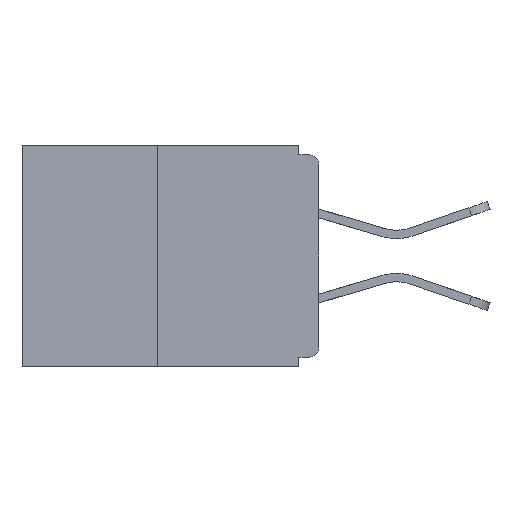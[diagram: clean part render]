
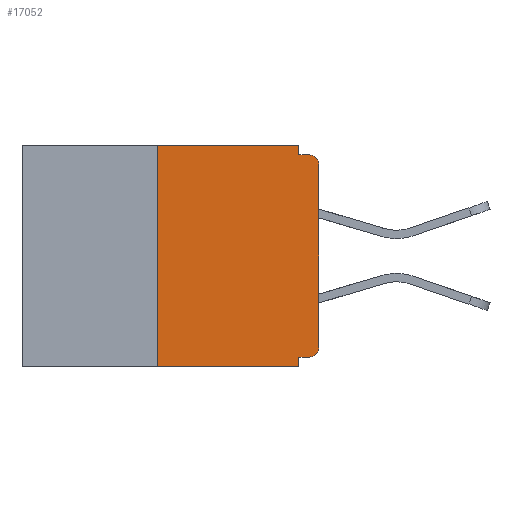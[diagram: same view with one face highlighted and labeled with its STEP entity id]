
A CAD part, left-side view. The second image highlights one B-rep face of the part: STEP entity #17052.
In plain terms, the highlighted planar face has unit normal (-1, 0, 0).
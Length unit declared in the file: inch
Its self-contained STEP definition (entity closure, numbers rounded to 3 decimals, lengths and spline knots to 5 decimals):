
#138 = EDGE_CURVE ( 'NONE', #7621, #7189, #15936, .T. ) ;
#241 = LINE ( 'NONE', #15287, #11779 ) ;
#291 = FACE_OUTER_BOUND ( 'NONE', #16553, .T. ) ;
#328 = CARTESIAN_POINT ( 'NONE',  ( 0., 0.46, -0.343 ) ) ;
#333 = DIRECTION ( 'NONE',  ( 0., 0., 1. ) ) ;
#506 = CIRCLE ( 'NONE', #9485, 0.015 ) ;
#1081 = CARTESIAN_POINT ( 'NONE',  ( 0., 0.46, 0. ) ) ;
#1442 = DIRECTION ( 'NONE',  ( -1., 0., 0. ) ) ;
#1635 = EDGE_CURVE ( 'NONE', #5819, #13735, #7759, .T. ) ;
#1679 = DIRECTION ( 'NONE',  ( 0., 0., -1. ) ) ;
#1821 = LINE ( 'NONE', #14050, #3307 ) ;
#2431 = EDGE_CURVE ( 'NONE', #8469, #7682, #3675, .T. ) ;
#2753 = ORIENTED_EDGE ( 'NONE', *, *, #8613, .T. ) ;
#3055 = CARTESIAN_POINT ( 'NONE',  ( 0., 0.015, -0.015 ) ) ;
#3108 = VECTOR ( 'NONE', #9096, 39.37008 ) ;
#3307 = VECTOR ( 'NONE', #333, 39.37008 ) ;
#3663 = CARTESIAN_POINT ( 'NONE',  ( 0., 0.015, -0.328 ) ) ;
#3675 = LINE ( 'NONE', #1081, #8158 ) ;
#3964 = CARTESIAN_POINT ( 'NONE',  ( 0., 0.031, -0.343 ) ) ;
#5098 = ORIENTED_EDGE ( 'NONE', *, *, #13063, .T. ) ;
#5332 = CARTESIAN_POINT ( 'NONE',  ( 0., 0.031, -0.015 ) ) ;
#5819 = VERTEX_POINT ( 'NONE', #5332 ) ;
#6394 = ORIENTED_EDGE ( 'NONE', *, *, #1635, .F. ) ;
#6465 = CARTESIAN_POINT ( 'NONE',  ( 0., 0.25, 0. ) ) ;
#7095 = DIRECTION ( 'NONE',  ( 0., 0., -1. ) ) ;
#7189 = VERTEX_POINT ( 'NONE', #10118 ) ;
#7287 = DIRECTION ( 'NONE',  ( 0., -1., 0. ) ) ;
#7350 = VERTEX_POINT ( 'NONE', #9395 ) ;
#7621 = VERTEX_POINT ( 'NONE', #3663 ) ;
#7682 = VERTEX_POINT ( 'NONE', #13269 ) ;
#7759 = LINE ( 'NONE', #12800, #9655 ) ;
#8140 = DIRECTION ( 'NONE',  ( 0., 0., -1. ) ) ;
#8158 = VECTOR ( 'NONE', #9282, 39.37008 ) ;
#8469 = VERTEX_POINT ( 'NONE', #6465 ) ;
#8613 = EDGE_CURVE ( 'NONE', #15337, #13735, #506, .T. ) ;
#8953 = ORIENTED_EDGE ( 'NONE', *, *, #14622, .F. ) ;
#9038 = CARTESIAN_POINT ( 'NONE',  ( 0., 0., -0.328 ) ) ;
#9096 = DIRECTION ( 'NONE',  ( 0., 1., 0. ) ) ;
#9282 = DIRECTION ( 'NONE',  ( 0., -1., 0. ) ) ;
#9342 = DIRECTION ( 'NONE',  ( 0., 0., -1. ) ) ;
#9395 = CARTESIAN_POINT ( 'NONE',  ( 0., 0., -0.313 ) ) ;
#9485 = AXIS2_PLACEMENT_3D ( 'NONE', #12541, #1442, #16675 ) ;
#9655 = VECTOR ( 'NONE', #7287, 39.37008 ) ;
#10040 = EDGE_CURVE ( 'NONE', #7682, #5819, #241, .T. ) ;
#10114 = ORIENTED_EDGE ( 'NONE', *, *, #14335, .T. ) ;
#10118 = CARTESIAN_POINT ( 'NONE',  ( 0., 0.031, -0.328 ) ) ;
#10811 = LINE ( 'NONE', #3964, #17464 ) ;
#11029 = VECTOR ( 'NONE', #12617, 39.37008 ) ;
#11166 = PLANE ( 'NONE',  #16465 ) ;
#11359 = CARTESIAN_POINT ( 'NONE',  ( 0., 0.46, 0. ) ) ;
#11487 = VECTOR ( 'NONE', #16562, 39.37008 ) ;
#11779 = VECTOR ( 'NONE', #7095, 39.37008 ) ;
#11919 = LINE ( 'NONE', #13744, #11487 ) ;
#12062 = CARTESIAN_POINT ( 'NONE',  ( 0., 0.015, -0.313 ) ) ;
#12153 = CARTESIAN_POINT ( 'NONE',  ( 0., 0., -0.03 ) ) ;
#12199 = CARTESIAN_POINT ( 'NONE',  ( 0., 0.031, -0.343 ) ) ;
#12541 = CARTESIAN_POINT ( 'NONE',  ( 0., 0.015, -0.03 ) ) ;
#12617 = DIRECTION ( 'NONE',  ( 0., -1., 0. ) ) ;
#12671 = ORIENTED_EDGE ( 'NONE', *, *, #13779, .T. ) ;
#12800 = CARTESIAN_POINT ( 'NONE',  ( 0., 0., -0.015 ) ) ;
#12835 = VERTEX_POINT ( 'NONE', #17239 ) ;
#13063 = EDGE_CURVE ( 'NONE', #7350, #15337, #11919, .T. ) ;
#13256 = VERTEX_POINT ( 'NONE', #12199 ) ;
#13269 = CARTESIAN_POINT ( 'NONE',  ( 0., 0.031, 0. ) ) ;
#13486 = EDGE_CURVE ( 'NONE', #7189, #13256, #10811, .T. ) ;
#13597 = ORIENTED_EDGE ( 'NONE', *, *, #13486, .F. ) ;
#13735 = VERTEX_POINT ( 'NONE', #3055 ) ;
#13744 = CARTESIAN_POINT ( 'NONE',  ( 0., 0., 0. ) ) ;
#13779 = EDGE_CURVE ( 'NONE', #12835, #13256, #16593, .T. ) ;
#14050 = CARTESIAN_POINT ( 'NONE',  ( 0., 0.25, 0. ) ) ;
#14335 = EDGE_CURVE ( 'NONE', #7621, #7350, #17659, .T. ) ;
#14362 = AXIS2_PLACEMENT_3D ( 'NONE', #12062, #16187, #9342 ) ;
#14531 = ORIENTED_EDGE ( 'NONE', *, *, #10040, .F. ) ;
#14622 = EDGE_CURVE ( 'NONE', #12835, #8469, #1821, .T. ) ;
#14850 = ORIENTED_EDGE ( 'NONE', *, *, #2431, .F. ) ;
#15287 = CARTESIAN_POINT ( 'NONE',  ( 0., 0.031, 0. ) ) ;
#15337 = VERTEX_POINT ( 'NONE', #12153 ) ;
#15936 = LINE ( 'NONE', #9038, #3108 ) ;
#16187 = DIRECTION ( 'NONE',  ( -1., 0., 0. ) ) ;
#16465 = AXIS2_PLACEMENT_3D ( 'NONE', #11359, #16734, #1679 ) ;
#16553 = EDGE_LOOP ( 'NONE', ( #14850, #8953, #12671, #13597, #17615, #10114, #5098, #2753, #6394, #14531 ) ) ;
#16562 = DIRECTION ( 'NONE',  ( 0., 0., 1. ) ) ;
#16593 = LINE ( 'NONE', #328, #11029 ) ;
#16675 = DIRECTION ( 'NONE',  ( 0., 0., -1. ) ) ;
#16734 = DIRECTION ( 'NONE',  ( 1., 0., 0. ) ) ;
#17052 = ADVANCED_FACE ( 'NONE', ( #291 ), #11166, .F. ) ;
#17239 = CARTESIAN_POINT ( 'NONE',  ( 0., 0.25, -0.343 ) ) ;
#17464 = VECTOR ( 'NONE', #8140, 39.37008 ) ;
#17615 = ORIENTED_EDGE ( 'NONE', *, *, #138, .F. ) ;
#17659 = CIRCLE ( 'NONE', #14362, 0.015 ) ;
